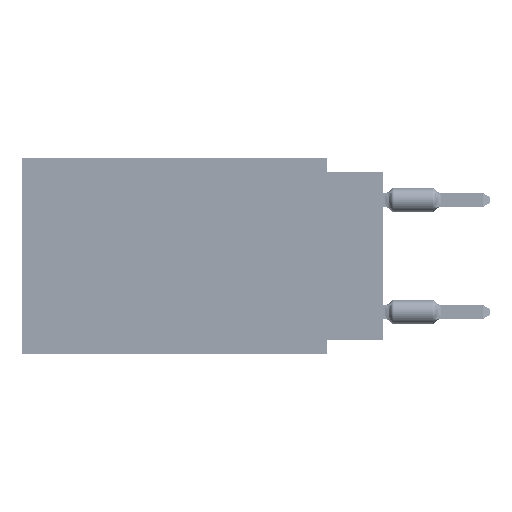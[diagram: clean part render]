
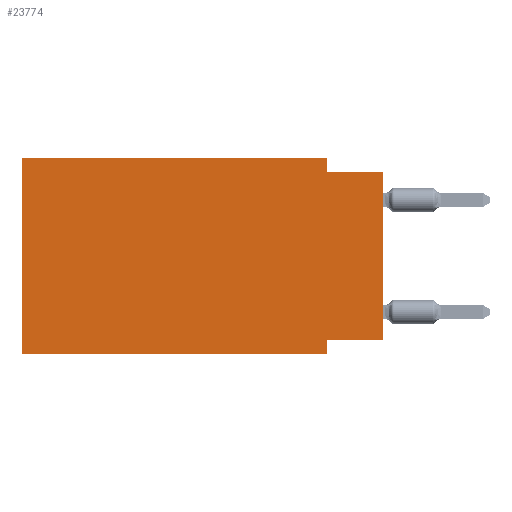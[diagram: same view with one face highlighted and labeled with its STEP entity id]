
A CAD part, left-side view. The second image highlights one B-rep face of the part: STEP entity #23774.
In plain terms, the highlighted planar face has unit normal (-1, 0, 0).
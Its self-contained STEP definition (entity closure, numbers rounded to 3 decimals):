
#535 = VECTOR ( 'NONE', #32796, 1000. ) ;
#2346 = LINE ( 'NONE', #43140, #34790 ) ;
#2689 = EDGE_CURVE ( 'NONE', #29206, #27466, #46238, .T. ) ;
#2925 = LINE ( 'NONE', #8397, #30368 ) ;
#3519 = DIRECTION ( 'NONE',  ( 0., 0., -1. ) ) ;
#3632 = CARTESIAN_POINT ( 'NONE',  ( 0., 16.383, 0. ) ) ;
#3776 = LINE ( 'NONE', #7745, #40159 ) ;
#7745 = CARTESIAN_POINT ( 'NONE',  ( 0., 16.383, -8.89 ) ) ;
#8397 = CARTESIAN_POINT ( 'NONE',  ( 0., 2.54, -8.89 ) ) ;
#9131 = CARTESIAN_POINT ( 'NONE',  ( 0., 0., 0. ) ) ;
#9579 = AXIS2_PLACEMENT_3D ( 'NONE', #57575, #49303, #29859 ) ;
#12701 = ORIENTED_EDGE ( 'NONE', *, *, #16698, .F. ) ;
#16544 = ORIENTED_EDGE ( 'NONE', *, *, #45989, .T. ) ;
#16698 = EDGE_CURVE ( 'NONE', #33891, #24752, #2925, .T. ) ;
#17501 = CARTESIAN_POINT ( 'NONE',  ( 0., 2.54, 0. ) ) ;
#17833 = EDGE_LOOP ( 'NONE', ( #34032, #29290, #26868, #56689, #22602, #16544, #12701, #36884 ) ) ;
#18655 = CARTESIAN_POINT ( 'NONE',  ( 0., 2.54, -8.89 ) ) ;
#19327 = LINE ( 'NONE', #34500, #55811 ) ;
#19423 = CARTESIAN_POINT ( 'NONE',  ( 0., 2.54, -0.635 ) ) ;
#19629 = DIRECTION ( 'NONE',  ( 0., 0., -1. ) ) ;
#21329 = VERTEX_POINT ( 'NONE', #17501 ) ;
#22602 = ORIENTED_EDGE ( 'NONE', *, *, #32617, .F. ) ;
#22972 = VERTEX_POINT ( 'NONE', #3632 ) ;
#23774 = ADVANCED_FACE ( 'NONE', ( #30161 ), #38983, .F. ) ;
#23901 = EDGE_CURVE ( 'NONE', #57147, #27466, #50206, .T. ) ;
#24752 = VERTEX_POINT ( 'NONE', #18655 ) ;
#24805 = VECTOR ( 'NONE', #28275, 1000. ) ;
#26868 = ORIENTED_EDGE ( 'NONE', *, *, #31079, .F. ) ;
#27082 = DIRECTION ( 'NONE',  ( 0., 0., 1. ) ) ;
#27466 = VERTEX_POINT ( 'NONE', #54517 ) ;
#28275 = DIRECTION ( 'NONE',  ( 0., -1., 0. ) ) ;
#29206 = VERTEX_POINT ( 'NONE', #19423 ) ;
#29235 = CARTESIAN_POINT ( 'NONE',  ( 0., 2.54, -8.255 ) ) ;
#29290 = ORIENTED_EDGE ( 'NONE', *, *, #2689, .F. ) ;
#29859 = DIRECTION ( 'NONE',  ( 0., 0., -1. ) ) ;
#30161 = FACE_OUTER_BOUND ( 'NONE', #17833, .T. ) ;
#30368 = VECTOR ( 'NONE', #3519, 1000. ) ;
#30704 = VERTEX_POINT ( 'NONE', #56353 ) ;
#31079 = EDGE_CURVE ( 'NONE', #21329, #29206, #51298, .T. ) ;
#32231 = CARTESIAN_POINT ( 'NONE',  ( 0., 0., -0.635 ) ) ;
#32617 = EDGE_CURVE ( 'NONE', #30704, #22972, #33702, .T. ) ;
#32796 = DIRECTION ( 'NONE',  ( 0., 0., 1. ) ) ;
#33702 = LINE ( 'NONE', #43109, #535 ) ;
#33891 = VERTEX_POINT ( 'NONE', #29235 ) ;
#34032 = ORIENTED_EDGE ( 'NONE', *, *, #23901, .T. ) ;
#34500 = CARTESIAN_POINT ( 'NONE',  ( 0., 0., -8.255 ) ) ;
#34790 = VECTOR ( 'NONE', #48006, 1000. ) ;
#34846 = VECTOR ( 'NONE', #27082, 1000. ) ;
#36442 = CARTESIAN_POINT ( 'NONE',  ( 0., 0., -8.255 ) ) ;
#36884 = ORIENTED_EDGE ( 'NONE', *, *, #58938, .F. ) ;
#38772 = DIRECTION ( 'NONE',  ( 0., 1., 0. ) ) ;
#38983 = PLANE ( 'NONE',  #9579 ) ;
#40159 = VECTOR ( 'NONE', #40610, 1000. ) ;
#40610 = DIRECTION ( 'NONE',  ( 0., -1., 0. ) ) ;
#43109 = CARTESIAN_POINT ( 'NONE',  ( 0., 16.383, 0. ) ) ;
#43140 = CARTESIAN_POINT ( 'NONE',  ( 0., 16.383, 0. ) ) ;
#43141 = VECTOR ( 'NONE', #19629, 1000. ) ;
#45989 = EDGE_CURVE ( 'NONE', #30704, #24752, #3776, .T. ) ;
#46238 = LINE ( 'NONE', #32231, #24805 ) ;
#47319 = CARTESIAN_POINT ( 'NONE',  ( 0., 2.54, 0. ) ) ;
#48006 = DIRECTION ( 'NONE',  ( 0., -1., 0. ) ) ;
#49303 = DIRECTION ( 'NONE',  ( 1., 0., 0. ) ) ;
#50206 = LINE ( 'NONE', #9131, #34846 ) ;
#51298 = LINE ( 'NONE', #47319, #43141 ) ;
#51986 = EDGE_CURVE ( 'NONE', #22972, #21329, #2346, .T. ) ;
#54517 = CARTESIAN_POINT ( 'NONE',  ( 0., 0., -0.635 ) ) ;
#55811 = VECTOR ( 'NONE', #38772, 1000. ) ;
#56353 = CARTESIAN_POINT ( 'NONE',  ( 0., 16.383, -8.89 ) ) ;
#56689 = ORIENTED_EDGE ( 'NONE', *, *, #51986, .F. ) ;
#57147 = VERTEX_POINT ( 'NONE', #36442 ) ;
#57575 = CARTESIAN_POINT ( 'NONE',  ( 0., 16.383, 0. ) ) ;
#58938 = EDGE_CURVE ( 'NONE', #57147, #33891, #19327, .T. ) ;
